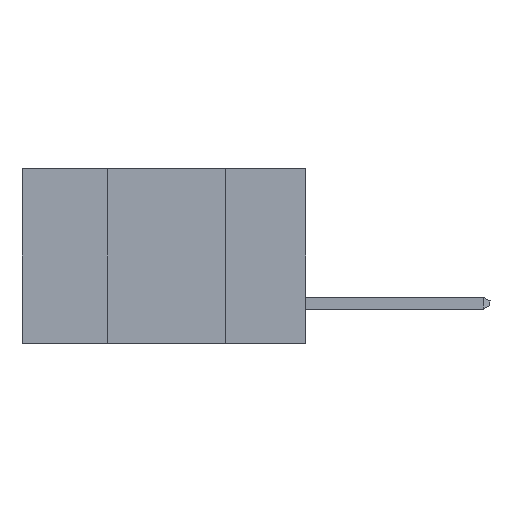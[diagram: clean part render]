
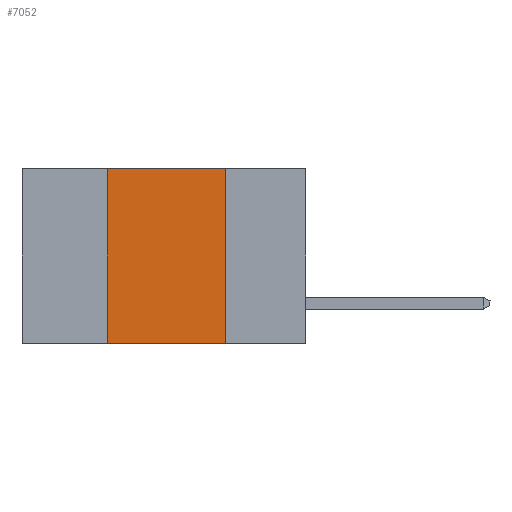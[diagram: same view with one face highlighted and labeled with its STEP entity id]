
A CAD part, left-side view. The second image highlights one B-rep face of the part: STEP entity #7052.
In plain terms, the highlighted planar face has unit normal (-1, 0, 0).
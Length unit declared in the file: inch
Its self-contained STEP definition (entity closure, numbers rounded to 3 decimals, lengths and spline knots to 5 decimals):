
#585 = VECTOR ( 'NONE', #8977, 39.37008 ) ;
#734 = AXIS2_PLACEMENT_3D ( 'NONE', #3654, #2146, #1215 ) ;
#918 = EDGE_CURVE ( 'NONE', #4600, #5557, #4746, .T. ) ;
#1215 = DIRECTION ( 'NONE',  ( 0., 0., -1. ) ) ;
#1354 = FACE_OUTER_BOUND ( 'NONE', #5582, .T. ) ;
#1407 = LINE ( 'NONE', #4455, #9736 ) ;
#1569 = ORIENTED_EDGE ( 'NONE', *, *, #7761, .T. ) ;
#2146 = DIRECTION ( 'NONE',  ( 1., 0., 0. ) ) ;
#2517 = ORIENTED_EDGE ( 'NONE', *, *, #9810, .F. ) ;
#2789 = CARTESIAN_POINT ( 'NONE',  ( 0., 0.17, 0. ) ) ;
#3654 = CARTESIAN_POINT ( 'NONE',  ( 0., 0.6, 0. ) ) ;
#3665 = VECTOR ( 'NONE', #3993, 39.37008 ) ;
#3993 = DIRECTION ( 'NONE',  ( 0., 0., -1. ) ) ;
#4039 = DIRECTION ( 'NONE',  ( 0., 0., 1. ) ) ;
#4455 = CARTESIAN_POINT ( 'NONE',  ( 0., 0.6, -0.37 ) ) ;
#4600 = VERTEX_POINT ( 'NONE', #2789 ) ;
#4746 = LINE ( 'NONE', #7820, #3665 ) ;
#4788 = LINE ( 'NONE', #7861, #5871 ) ;
#4920 = CARTESIAN_POINT ( 'NONE',  ( 0., 0.17, -0.37 ) ) ;
#5557 = VERTEX_POINT ( 'NONE', #4920 ) ;
#5582 = EDGE_LOOP ( 'NONE', ( #5884, #8265, #2517, #1569 ) ) ;
#5612 = CARTESIAN_POINT ( 'NONE',  ( 0., 0.42, 0. ) ) ;
#5776 = PLANE ( 'NONE',  #734 ) ;
#5860 = CARTESIAN_POINT ( 'NONE',  ( 0., 0.42, -0.37 ) ) ;
#5871 = VECTOR ( 'NONE', #4039, 39.37008 ) ;
#5884 = ORIENTED_EDGE ( 'NONE', *, *, #918, .F. ) ;
#5909 = LINE ( 'NONE', #8077, #585 ) ;
#7052 = ADVANCED_FACE ( 'NONE', ( #1354 ), #5776, .F. ) ;
#7761 = EDGE_CURVE ( 'NONE', #9468, #5557, #1407, .T. ) ;
#7820 = CARTESIAN_POINT ( 'NONE',  ( 0., 0.17, -0.37 ) ) ;
#7861 = CARTESIAN_POINT ( 'NONE',  ( 0., 0.42, -0.37 ) ) ;
#7882 = VERTEX_POINT ( 'NONE', #5612 ) ;
#8074 = EDGE_CURVE ( 'NONE', #7882, #4600, #5909, .T. ) ;
#8077 = CARTESIAN_POINT ( 'NONE',  ( 0., 0.6, 0. ) ) ;
#8265 = ORIENTED_EDGE ( 'NONE', *, *, #8074, .F. ) ;
#8977 = DIRECTION ( 'NONE',  ( 0., -1., 0. ) ) ;
#8989 = DIRECTION ( 'NONE',  ( 0., -1., 0. ) ) ;
#9468 = VERTEX_POINT ( 'NONE', #5860 ) ;
#9736 = VECTOR ( 'NONE', #8989, 39.37008 ) ;
#9810 = EDGE_CURVE ( 'NONE', #9468, #7882, #4788, .T. ) ;
